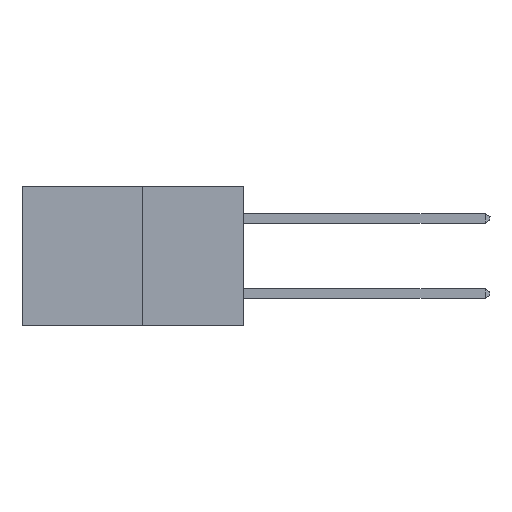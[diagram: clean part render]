
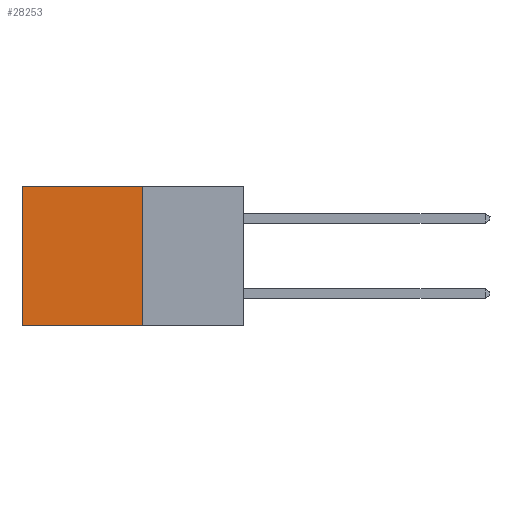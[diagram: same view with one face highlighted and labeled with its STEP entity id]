
A CAD part, left-side view. The second image highlights one B-rep face of the part: STEP entity #28253.
In plain terms, the highlighted planar face has unit normal (-1, 0, 0).
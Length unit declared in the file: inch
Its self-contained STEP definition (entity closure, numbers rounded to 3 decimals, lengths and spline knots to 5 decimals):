
#1256 = AXIS2_PLACEMENT_3D ( 'NONE', #20106, #4806, #22682 ) ;
#1370 = CARTESIAN_POINT ( 'NONE',  ( 0.277, 0.27, 0. ) ) ;
#1530 = ORIENTED_EDGE ( 'NONE', *, *, #3696, .F. ) ;
#3696 = EDGE_CURVE ( 'NONE', #7742, #16772, #28799, .T. ) ;
#4038 = DIRECTION ( 'NONE',  ( 0., 1., 0. ) ) ;
#4800 = LINE ( 'NONE', #19528, #31109 ) ;
#4806 = DIRECTION ( 'NONE',  ( 1., 0., 0. ) ) ;
#5200 = CARTESIAN_POINT ( 'NONE',  ( 0.277, 0.27, -0.37 ) ) ;
#7742 = VERTEX_POINT ( 'NONE', #30201 ) ;
#7873 = VECTOR ( 'NONE', #28235, 39.37008 ) ;
#8243 = LINE ( 'NONE', #1370, #27724 ) ;
#8498 = ORIENTED_EDGE ( 'NONE', *, *, #21657, .F. ) ;
#9735 = VERTEX_POINT ( 'NONE', #23953 ) ;
#9769 = EDGE_LOOP ( 'NONE', ( #23596, #8498, #1530, #23624 ) ) ;
#10472 = CARTESIAN_POINT ( 'NONE',  ( 0.277, 0.59, -0.37 ) ) ;
#12717 = FACE_OUTER_BOUND ( 'NONE', #9769, .T. ) ;
#15020 = PLANE ( 'NONE',  #1256 ) ;
#15167 = EDGE_CURVE ( 'NONE', #7742, #32976, #8243, .T. ) ;
#15294 = VECTOR ( 'NONE', #30622, 39.37008 ) ;
#16512 = CARTESIAN_POINT ( 'NONE',  ( 0.277, 0.59, 0. ) ) ;
#16772 = VERTEX_POINT ( 'NONE', #5200 ) ;
#19528 = CARTESIAN_POINT ( 'NONE',  ( 0.277, 0.27, -0.37 ) ) ;
#20106 = CARTESIAN_POINT ( 'NONE',  ( 0.277, 0.27, -0.37 ) ) ;
#21657 = EDGE_CURVE ( 'NONE', #16772, #9735, #4800, .T. ) ;
#22682 = DIRECTION ( 'NONE',  ( 0., 0., -1. ) ) ;
#23596 = ORIENTED_EDGE ( 'NONE', *, *, #31978, .T. ) ;
#23624 = ORIENTED_EDGE ( 'NONE', *, *, #15167, .T. ) ;
#23953 = CARTESIAN_POINT ( 'NONE',  ( 0.277, 0.59, -0.37 ) ) ;
#24752 = DIRECTION ( 'NONE',  ( 0., 1., 0. ) ) ;
#27724 = VECTOR ( 'NONE', #4038, 39.37008 ) ;
#28157 = LINE ( 'NONE', #10472, #7873 ) ;
#28235 = DIRECTION ( 'NONE',  ( 0., 0., -1. ) ) ;
#28253 = ADVANCED_FACE ( 'NONE', ( #12717 ), #15020, .F. ) ;
#28799 = LINE ( 'NONE', #30672, #15294 ) ;
#30201 = CARTESIAN_POINT ( 'NONE',  ( 0.277, 0.27, 0. ) ) ;
#30622 = DIRECTION ( 'NONE',  ( 0., 0., -1. ) ) ;
#30672 = CARTESIAN_POINT ( 'NONE',  ( 0.277, 0.27, -0.37 ) ) ;
#31109 = VECTOR ( 'NONE', #24752, 39.37008 ) ;
#31978 = EDGE_CURVE ( 'NONE', #32976, #9735, #28157, .T. ) ;
#32976 = VERTEX_POINT ( 'NONE', #16512 ) ;
